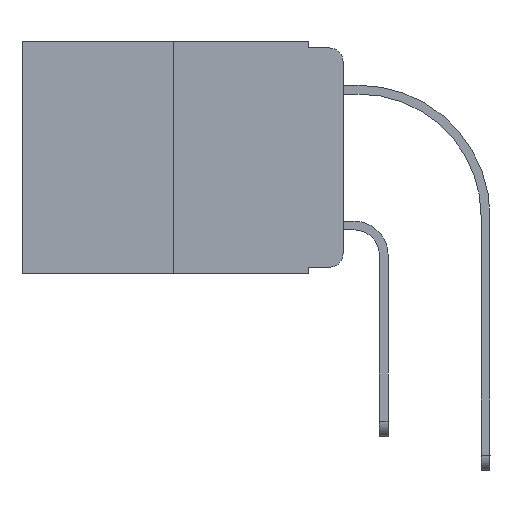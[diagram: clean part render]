
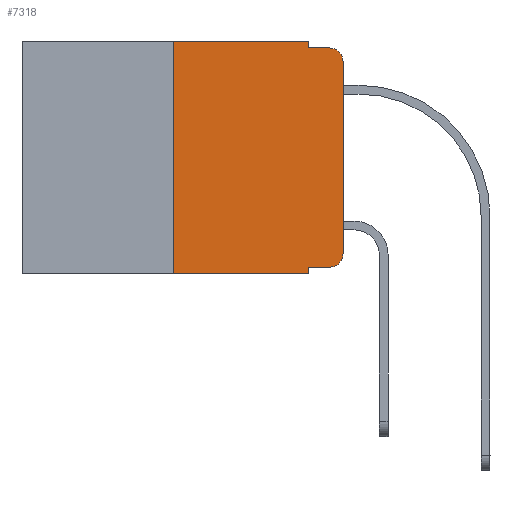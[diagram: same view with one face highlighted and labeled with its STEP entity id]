
A CAD part, left-side view. The second image highlights one B-rep face of the part: STEP entity #7318.
In plain terms, the highlighted planar face has unit normal (-1, 0, 0).
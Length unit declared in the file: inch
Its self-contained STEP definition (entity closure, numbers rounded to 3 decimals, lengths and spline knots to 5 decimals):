
#374 = DIRECTION ( 'NONE',  ( 0., -1., 0. ) ) ;
#572 = EDGE_CURVE ( 'NONE', #5117, #8574, #1917, .T. ) ;
#648 = LINE ( 'NONE', #6703, #4619 ) ;
#667 = EDGE_LOOP ( 'NONE', ( #8218, #11938, #8597, #9682, #9568, #1734, #10014, #3073, #3004, #1760 ) ) ;
#846 = VERTEX_POINT ( 'NONE', #8967 ) ;
#857 = EDGE_CURVE ( 'NONE', #12890, #5878, #5598, .T. ) ;
#944 = LINE ( 'NONE', #12954, #6626 ) ;
#1031 = EDGE_CURVE ( 'NONE', #4119, #6164, #12519, .T. ) ;
#1429 = CARTESIAN_POINT ( 'NONE',  ( 0., 0.02, -0.313 ) ) ;
#1639 = CARTESIAN_POINT ( 'NONE',  ( 0., 0.02, -0.01 ) ) ;
#1734 = ORIENTED_EDGE ( 'NONE', *, *, #8024, .F. ) ;
#1760 = ORIENTED_EDGE ( 'NONE', *, *, #7948, .T. ) ;
#1917 = LINE ( 'NONE', #5989, #8404 ) ;
#2215 = DIRECTION ( 'NONE',  ( -1., 0., 0. ) ) ;
#2223 = CARTESIAN_POINT ( 'NONE',  ( 0., 0.051, -0.333 ) ) ;
#2251 = PLANE ( 'NONE',  #10166 ) ;
#2345 = LINE ( 'NONE', #11541, #9891 ) ;
#2953 = VECTOR ( 'NONE', #8080, 39.37008 ) ;
#3004 = ORIENTED_EDGE ( 'NONE', *, *, #1031, .T. ) ;
#3073 = ORIENTED_EDGE ( 'NONE', *, *, #3447, .F. ) ;
#3192 = CARTESIAN_POINT ( 'NONE',  ( 0., 0.25, -0.343 ) ) ;
#3292 = VECTOR ( 'NONE', #374, 39.37008 ) ;
#3315 = CARTESIAN_POINT ( 'NONE',  ( 0., 0.473, 0. ) ) ;
#3397 = DIRECTION ( 'NONE',  ( 0., 0., -1. ) ) ;
#3447 = EDGE_CURVE ( 'NONE', #4119, #846, #2345, .T. ) ;
#3504 = DIRECTION ( 'NONE',  ( 0., -1., 0. ) ) ;
#3610 = DIRECTION ( 'NONE',  ( 0., 0., -1. ) ) ;
#3687 = DIRECTION ( 'NONE',  ( -1., 0., 0. ) ) ;
#3792 = DIRECTION ( 'NONE',  ( 0., -1., 0. ) ) ;
#3951 = DIRECTION ( 'NONE',  ( 0., 0., 1. ) ) ;
#4119 = VERTEX_POINT ( 'NONE', #2223 ) ;
#4619 = VECTOR ( 'NONE', #10809, 39.37008 ) ;
#5117 = VERTEX_POINT ( 'NONE', #12322 ) ;
#5199 = EDGE_CURVE ( 'NONE', #11045, #12890, #648, .T. ) ;
#5598 = LINE ( 'NONE', #11872, #10752 ) ;
#5878 = VERTEX_POINT ( 'NONE', #1639 ) ;
#5989 = CARTESIAN_POINT ( 'NONE',  ( 0., 0., 0. ) ) ;
#6164 = VERTEX_POINT ( 'NONE', #7647 ) ;
#6210 = AXIS2_PLACEMENT_3D ( 'NONE', #11363, #2215, #8256 ) ;
#6626 = VECTOR ( 'NONE', #3951, 39.37008 ) ;
#6703 = CARTESIAN_POINT ( 'NONE',  ( 0., 0.051, 0. ) ) ;
#6895 = VECTOR ( 'NONE', #3504, 39.37008 ) ;
#7273 = CIRCLE ( 'NONE', #6210, 0.02 ) ;
#7318 = ADVANCED_FACE ( 'NONE', ( #11518 ), #2251, .F. ) ;
#7400 = CARTESIAN_POINT ( 'NONE',  ( 0., 0.051, -0.333 ) ) ;
#7428 = EDGE_CURVE ( 'NONE', #8572, #11045, #12573, .T. ) ;
#7647 = CARTESIAN_POINT ( 'NONE',  ( 0., 0.02, -0.333 ) ) ;
#7948 = EDGE_CURVE ( 'NONE', #6164, #5117, #11334, .T. ) ;
#8024 = EDGE_CURVE ( 'NONE', #10838, #8572, #944, .T. ) ;
#8080 = DIRECTION ( 'NONE',  ( 0., -1., 0. ) ) ;
#8218 = ORIENTED_EDGE ( 'NONE', *, *, #572, .T. ) ;
#8256 = DIRECTION ( 'NONE',  ( 0., 0., -1. ) ) ;
#8404 = VECTOR ( 'NONE', #10066, 39.37008 ) ;
#8572 = VERTEX_POINT ( 'NONE', #9549 ) ;
#8574 = VERTEX_POINT ( 'NONE', #12313 ) ;
#8597 = ORIENTED_EDGE ( 'NONE', *, *, #857, .F. ) ;
#8753 = CARTESIAN_POINT ( 'NONE',  ( 0., 0.473, 0. ) ) ;
#8967 = CARTESIAN_POINT ( 'NONE',  ( 0., 0.051, -0.343 ) ) ;
#9192 = CARTESIAN_POINT ( 'NONE',  ( 0., 0.473, -0.343 ) ) ;
#9345 = DIRECTION ( 'NONE',  ( 0., 0., -1. ) ) ;
#9422 = EDGE_CURVE ( 'NONE', #8574, #5878, #7273, .T. ) ;
#9542 = CARTESIAN_POINT ( 'NONE',  ( 0., 0.051, -0.01 ) ) ;
#9549 = CARTESIAN_POINT ( 'NONE',  ( 0., 0.25, 0. ) ) ;
#9568 = ORIENTED_EDGE ( 'NONE', *, *, #7428, .F. ) ;
#9682 = ORIENTED_EDGE ( 'NONE', *, *, #5199, .F. ) ;
#9891 = VECTOR ( 'NONE', #3397, 39.37008 ) ;
#10014 = ORIENTED_EDGE ( 'NONE', *, *, #13071, .T. ) ;
#10066 = DIRECTION ( 'NONE',  ( 0., 0., 1. ) ) ;
#10166 = AXIS2_PLACEMENT_3D ( 'NONE', #3315, #11266, #9345 ) ;
#10752 = VECTOR ( 'NONE', #3792, 39.37008 ) ;
#10809 = DIRECTION ( 'NONE',  ( 0., 0., -1. ) ) ;
#10838 = VERTEX_POINT ( 'NONE', #3192 ) ;
#11045 = VERTEX_POINT ( 'NONE', #12842 ) ;
#11266 = DIRECTION ( 'NONE',  ( 1., 0., 0. ) ) ;
#11309 = LINE ( 'NONE', #9192, #2953 ) ;
#11334 = CIRCLE ( 'NONE', #12377, 0.02 ) ;
#11363 = CARTESIAN_POINT ( 'NONE',  ( 0., 0.02, -0.03 ) ) ;
#11518 = FACE_OUTER_BOUND ( 'NONE', #667, .T. ) ;
#11541 = CARTESIAN_POINT ( 'NONE',  ( 0., 0.051, 0. ) ) ;
#11872 = CARTESIAN_POINT ( 'NONE',  ( 0., 0.051, -0.01 ) ) ;
#11938 = ORIENTED_EDGE ( 'NONE', *, *, #9422, .T. ) ;
#12313 = CARTESIAN_POINT ( 'NONE',  ( 0., 0., -0.03 ) ) ;
#12322 = CARTESIAN_POINT ( 'NONE',  ( 0., 0., -0.313 ) ) ;
#12377 = AXIS2_PLACEMENT_3D ( 'NONE', #1429, #3687, #3610 ) ;
#12519 = LINE ( 'NONE', #7400, #6895 ) ;
#12573 = LINE ( 'NONE', #8753, #3292 ) ;
#12842 = CARTESIAN_POINT ( 'NONE',  ( 0., 0.051, 0. ) ) ;
#12890 = VERTEX_POINT ( 'NONE', #9542 ) ;
#12954 = CARTESIAN_POINT ( 'NONE',  ( 0., 0.25, 0. ) ) ;
#13071 = EDGE_CURVE ( 'NONE', #10838, #846, #11309, .T. ) ;
